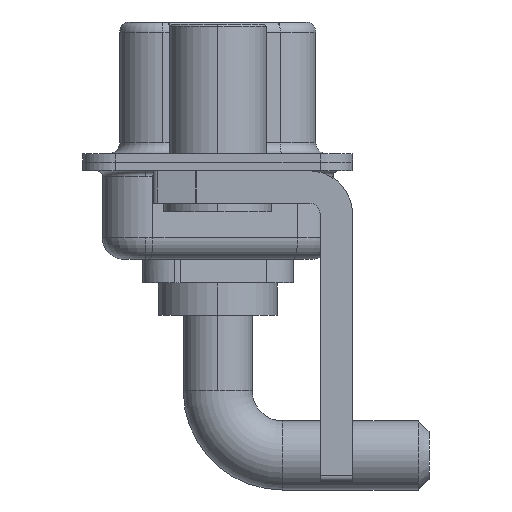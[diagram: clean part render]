
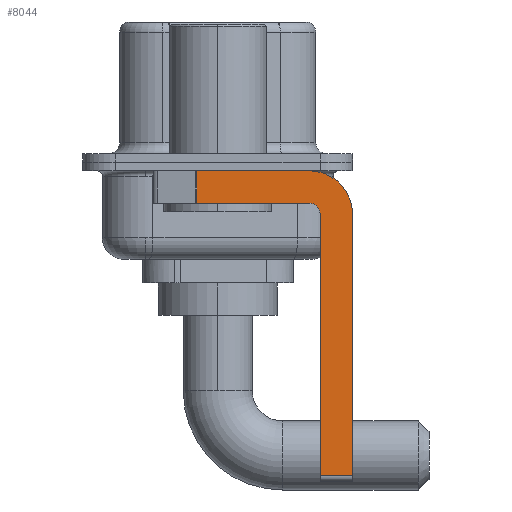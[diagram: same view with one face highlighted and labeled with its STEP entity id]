
A CAD part, left-side view. The second image highlights one B-rep face of the part: STEP entity #8044.
In plain terms, the highlighted planar face has unit normal (-1, 0, 0).
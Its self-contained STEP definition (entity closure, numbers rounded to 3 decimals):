
#273 = ORIENTED_EDGE ( 'NONE', *, *, #15919, .F. ) ;
#323 = CARTESIAN_POINT ( 'NONE',  ( -2.9, -4.25, -0.4 ) ) ;
#551 = DIRECTION ( 'NONE',  ( 0., 0., 1. ) ) ;
#1012 = CARTESIAN_POINT ( 'NONE',  ( -2.9, 0.978, -1.9 ) ) ;
#1115 = ORIENTED_EDGE ( 'NONE', *, *, #16008, .T. ) ;
#1669 = DIRECTION ( 'NONE',  ( 0., 0., 1. ) ) ;
#1748 = EDGE_CURVE ( 'NONE', #14542, #9101, #5475, .T. ) ;
#1799 = VERTEX_POINT ( 'NONE', #2590 ) ;
#2039 = CARTESIAN_POINT ( 'NONE',  ( -2.9, -4.25, -2.4 ) ) ;
#2337 = VECTOR ( 'NONE', #9554, 1000. ) ;
#2386 = CIRCLE ( 'NONE', #11984, 0.5 ) ;
#2590 = CARTESIAN_POINT ( 'NONE',  ( -2.9, -4.25, -1.9 ) ) ;
#3335 = DIRECTION ( 'NONE',  ( 1., 0., 0. ) ) ;
#3784 = ORIENTED_EDGE ( 'NONE', *, *, #5606, .F. ) ;
#4247 = ORIENTED_EDGE ( 'NONE', *, *, #15856, .F. ) ;
#4555 = VERTEX_POINT ( 'NONE', #16772 ) ;
#4835 = DIRECTION ( 'NONE',  ( 0., 0., -1. ) ) ;
#4921 = LINE ( 'NONE', #7579, #12239 ) ;
#5353 = PLANE ( 'NONE',  #8351 ) ;
#5475 = LINE ( 'NONE', #1012, #2337 ) ;
#5606 = EDGE_CURVE ( 'NONE', #14542, #16930, #10513, .T. ) ;
#5699 = DIRECTION ( 'NONE',  ( 0., 1., 0. ) ) ;
#5793 = CARTESIAN_POINT ( 'NONE',  ( -2.9, -4.25, -1.9 ) ) ;
#6581 = CARTESIAN_POINT ( 'NONE',  ( -2.9, -4.25, -2.4 ) ) ;
#7397 = DIRECTION ( 'NONE',  ( -1., 0., 0. ) ) ;
#7579 = CARTESIAN_POINT ( 'NONE',  ( -2.9, -4.25, -14.55 ) ) ;
#7624 = ORIENTED_EDGE ( 'NONE', *, *, #9233, .F. ) ;
#7999 = FACE_OUTER_BOUND ( 'NONE', #18362, .T. ) ;
#8044 = ADVANCED_FACE ( 'NONE', ( #7999 ), #5353, .F. ) ;
#8351 = AXIS2_PLACEMENT_3D ( 'NONE', #6581, #13741, #18372 ) ;
#8436 = LINE ( 'NONE', #5793, #15181 ) ;
#9014 = ORIENTED_EDGE ( 'NONE', *, *, #1748, .T. ) ;
#9101 = VERTEX_POINT ( 'NONE', #18040 ) ;
#9177 = CARTESIAN_POINT ( 'NONE',  ( -2.9, -4.25, -2.4 ) ) ;
#9233 = EDGE_CURVE ( 'NONE', #15992, #12124, #17089, .T. ) ;
#9554 = DIRECTION ( 'NONE',  ( 0., 0., -1. ) ) ;
#10219 = CARTESIAN_POINT ( 'NONE',  ( -2.9, -4.75, -14.8 ) ) ;
#10308 = DIRECTION ( 'NONE',  ( 0., -1., 0. ) ) ;
#10415 = VECTOR ( 'NONE', #1669, 1000. ) ;
#10432 = AXIS2_PLACEMENT_3D ( 'NONE', #2039, #3335, #4835 ) ;
#10495 = CARTESIAN_POINT ( 'NONE',  ( -2.9, -6.25, -2.4 ) ) ;
#10513 = LINE ( 'NONE', #16353, #13108 ) ;
#11902 = EDGE_CURVE ( 'NONE', #1799, #9101, #8436, .T. ) ;
#11984 = AXIS2_PLACEMENT_3D ( 'NONE', #9177, #7397, #551 ) ;
#12124 = VERTEX_POINT ( 'NONE', #14658 ) ;
#12239 = VECTOR ( 'NONE', #10308, 1000. ) ;
#12947 = LINE ( 'NONE', #10219, #10415 ) ;
#13108 = VECTOR ( 'NONE', #17859, 1000. ) ;
#13403 = CARTESIAN_POINT ( 'NONE',  ( -2.9, 0.978, -0.4 ) ) ;
#13625 = ORIENTED_EDGE ( 'NONE', *, *, #17513, .F. ) ;
#13741 = DIRECTION ( 'NONE',  ( 1., 0., 0. ) ) ;
#14318 = VERTEX_POINT ( 'NONE', #15308 ) ;
#14440 = CARTESIAN_POINT ( 'NONE',  ( -2.9, -6.25, -2.4 ) ) ;
#14542 = VERTEX_POINT ( 'NONE', #13403 ) ;
#14658 = CARTESIAN_POINT ( 'NONE',  ( -2.9, -6.25, -14.55 ) ) ;
#15181 = VECTOR ( 'NONE', #5699, 1000. ) ;
#15308 = CARTESIAN_POINT ( 'NONE',  ( -2.9, -4.75, -14.55 ) ) ;
#15856 = EDGE_CURVE ( 'NONE', #14318, #4555, #12947, .T. ) ;
#15919 = EDGE_CURVE ( 'NONE', #16930, #15992, #18570, .T. ) ;
#15960 = DIRECTION ( 'NONE',  ( 0., 0., -1. ) ) ;
#15992 = VERTEX_POINT ( 'NONE', #10495 ) ;
#16008 = EDGE_CURVE ( 'NONE', #14318, #12124, #4921, .T. ) ;
#16353 = CARTESIAN_POINT ( 'NONE',  ( -2.9, 3., -0.4 ) ) ;
#16772 = CARTESIAN_POINT ( 'NONE',  ( -2.9, -4.75, -2.4 ) ) ;
#16920 = VECTOR ( 'NONE', #15960, 1000. ) ;
#16930 = VERTEX_POINT ( 'NONE', #323 ) ;
#17089 = LINE ( 'NONE', #14440, #16920 ) ;
#17513 = EDGE_CURVE ( 'NONE', #4555, #1799, #2386, .T. ) ;
#17859 = DIRECTION ( 'NONE',  ( 0., -1., 0. ) ) ;
#18040 = CARTESIAN_POINT ( 'NONE',  ( -2.9, 0.978, -1.9 ) ) ;
#18219 = ORIENTED_EDGE ( 'NONE', *, *, #11902, .F. ) ;
#18362 = EDGE_LOOP ( 'NONE', ( #3784, #9014, #18219, #13625, #4247, #1115, #7624, #273 ) ) ;
#18372 = DIRECTION ( 'NONE',  ( 0., 0., -1. ) ) ;
#18570 = CIRCLE ( 'NONE', #10432, 2. ) ;
